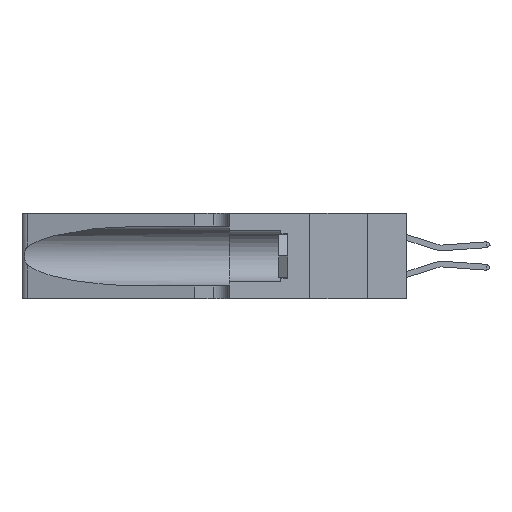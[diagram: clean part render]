
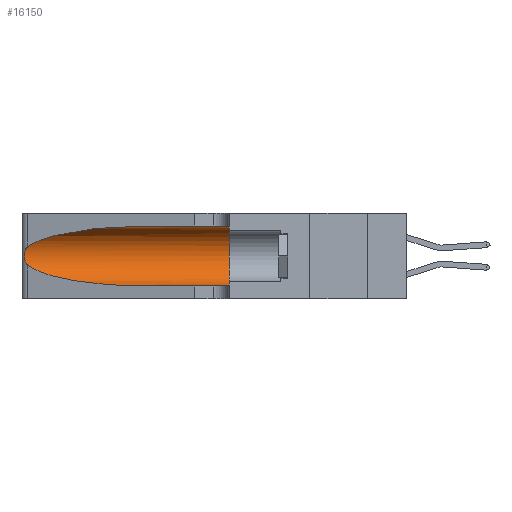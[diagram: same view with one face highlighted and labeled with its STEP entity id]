
A CAD part, left-side view. The second image highlights one B-rep face of the part: STEP entity #16150.
In plain terms, the highlighted cylindrical face has radius 3.308 mm (diameter 6.617 mm), a partial arc.
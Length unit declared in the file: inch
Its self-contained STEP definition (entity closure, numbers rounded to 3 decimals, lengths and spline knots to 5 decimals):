
#486 = ORIENTED_EDGE ( 'NONE', *, *, #4844, .T. ) ;
#889 = EDGE_CURVE ( 'NONE', #10362, #20176, #16285, .T. ) ;
#1071 = CARTESIAN_POINT ( 'NONE',  ( 0.26017, 1.23833, 0.17102 ) ) ;
#1486 = CYLINDRICAL_SURFACE ( 'NONE', #14618, 0.13025 ) ;
#2495 = CARTESIAN_POINT ( 'NONE',  ( 0.25639, 1.23184, 0.21858 ) ) ;
#2508 = CARTESIAN_POINT ( 'NONE',  ( 0.25487, 1.22718, 0.22369 ) ) ;
#2579 = VERTEX_POINT ( 'NONE', #3235 ) ;
#2772 = ORIENTED_EDGE ( 'NONE', *, *, #13080, .F. ) ;
#3235 = CARTESIAN_POINT ( 'NONE',  ( 0.25487, 1.22718, 0.14631 ) ) ;
#3304 = CARTESIAN_POINT ( 'NONE',  ( 0.1305, 0.72297, 0.31525 ) ) ;
#3445 = CARTESIAN_POINT ( 'NONE',  ( 0.1305, 1.61858, 0.31525 ) ) ;
#4004 = CARTESIAN_POINT ( 'NONE',  ( 0.25789, 1.23486, 0.15765 ) ) ;
#4145 = CARTESIAN_POINT ( 'NONE',  ( 0.25487, 1.22718, 0.22369 ) ) ;
#4205 = B_SPLINE_CURVE_WITH_KNOTS ( 'NONE', 3,
 ( #4145, #8917, #2495, #18346, #7298, #16815, #7151, #19800, #1071, #13548, #4004, #10440, #20000, #8844 ),
 .UNSPECIFIED., .F., .F.,
 ( 4, 2, 2, 2, 2, 2, 4 ),
 ( 0., 0.00027, 0.00053, 0.00107, 0.0016, 0.00187, 0.00214 ),
 .UNSPECIFIED. ) ;
#4394 = EDGE_CURVE ( 'NONE', #6285, #2579, #4205, .T. ) ;
#4625 = DIRECTION ( 'NONE',  ( 0., -1., 0. ) ) ;
#4844 = EDGE_CURVE ( 'NONE', #2579, #10362, #9988, .T. ) ;
#5320 = DIRECTION ( 'NONE',  ( 0., 1., 0. ) ) ;
#5375 = VECTOR ( 'NONE', #14432, 39.37008 ) ;
#6285 = VERTEX_POINT ( 'NONE', #2508 ) ;
#6297 =( BOUNDED_CURVE ( )  B_SPLINE_CURVE ( 3, ( #11094, #17352, #12488, #7929 ),
 .UNSPECIFIED., .F., .T. ) 
 B_SPLINE_CURVE_WITH_KNOTS ( ( 4, 4 ),
 ( 1.5708, 2.84003 ),
 .UNSPECIFIED. ) 
 CURVE ( )  GEOMETRIC_REPRESENTATION_ITEM ( )  RATIONAL_B_SPLINE_CURVE ( ( 1., 0.87, 0.87, 1. ) ) 
 REPRESENTATION_ITEM ( '' )  );
#7131 = DIRECTION ( 'NONE',  ( 0., 0., 1. ) ) ;
#7151 = CARTESIAN_POINT ( 'NONE',  ( 0.26075, 1.23896, 0.19203 ) ) ;
#7298 = CARTESIAN_POINT ( 'NONE',  ( 0.25854, 1.2359, 0.20912 ) ) ;
#7868 = CARTESIAN_POINT ( 'NONE',  ( 0.1305, 1.61858, 0.185 ) ) ;
#7929 = CARTESIAN_POINT ( 'NONE',  ( 0.25487, 1.22718, 0.22369 ) ) ;
#8217 = CARTESIAN_POINT ( 'NONE',  ( 0.1305, 0.72297, 0.05475 ) ) ;
#8728 = CARTESIAN_POINT ( 'NONE',  ( 0.25487, 1.22718, 0.14631 ) ) ;
#8844 = CARTESIAN_POINT ( 'NONE',  ( 0.25487, 1.22718, 0.14631 ) ) ;
#8917 = CARTESIAN_POINT ( 'NONE',  ( 0.25555, 1.22994, 0.2215 ) ) ;
#9678 = VERTEX_POINT ( 'NONE', #3304 ) ;
#9891 = EDGE_CURVE ( 'NONE', #9678, #10650, #12281, .T. ) ;
#9988 =( BOUNDED_CURVE ( )  B_SPLINE_CURVE ( 3, ( #8728, #14721, #14500, #8217 ),
 .UNSPECIFIED., .F., .T. ) 
 B_SPLINE_CURVE_WITH_KNOTS ( ( 4, 4 ),
 ( 3.44316, 4.71239 ),
 .UNSPECIFIED. ) 
 CURVE ( )  GEOMETRIC_REPRESENTATION_ITEM ( )  RATIONAL_B_SPLINE_CURVE ( ( 1., 0.87, 0.87, 1. ) ) 
 REPRESENTATION_ITEM ( '' )  );
#10362 = VERTEX_POINT ( 'NONE', #11983 ) ;
#10440 = CARTESIAN_POINT ( 'NONE',  ( 0.25639, 1.23186, 0.15144 ) ) ;
#10650 = VERTEX_POINT ( 'NONE', #20354 ) ;
#11094 = CARTESIAN_POINT ( 'NONE',  ( 0.1305, 0.72297, 0.31525 ) ) ;
#11978 = ORIENTED_EDGE ( 'NONE', *, *, #889, .T. ) ;
#11983 = CARTESIAN_POINT ( 'NONE',  ( 0.1305, 0.72297, 0.05475 ) ) ;
#12281 = LINE ( 'NONE', #3445, #5375 ) ;
#12450 = ORIENTED_EDGE ( 'NONE', *, *, #4394, .T. ) ;
#12488 = CARTESIAN_POINT ( 'NONE',  ( 0.2373, 1.15595, 0.28018 ) ) ;
#12538 = ORIENTED_EDGE ( 'NONE', *, *, #16108, .T. ) ;
#12758 = FACE_OUTER_BOUND ( 'NONE', #15875, .T. ) ;
#13080 = EDGE_CURVE ( 'NONE', #10650, #20176, #16396, .T. ) ;
#13085 = ORIENTED_EDGE ( 'NONE', *, *, #9891, .F. ) ;
#13168 = CARTESIAN_POINT ( 'NONE',  ( 0.1305, 0.35, 0.185 ) ) ;
#13548 = CARTESIAN_POINT ( 'NONE',  ( 0.25856, 1.23593, 0.16098 ) ) ;
#14432 = DIRECTION ( 'NONE',  ( 0., -1., 0. ) ) ;
#14500 = CARTESIAN_POINT ( 'NONE',  ( 0.18966, 0.96281, 0.05475 ) ) ;
#14618 = AXIS2_PLACEMENT_3D ( 'NONE', #7868, #4625, #15885 ) ;
#14721 = CARTESIAN_POINT ( 'NONE',  ( 0.2373, 1.15595, 0.08982 ) ) ;
#15875 = EDGE_LOOP ( 'NONE', ( #12538, #12450, #486, #11978, #2772, #13085 ) ) ;
#15885 = DIRECTION ( 'NONE',  ( 0., 0., -1. ) ) ;
#16108 = EDGE_CURVE ( 'NONE', #9678, #6285, #6297, .T. ) ;
#16150 = ADVANCED_FACE ( 'NONE', ( #12758 ), #1486, .F. ) ;
#16285 = LINE ( 'NONE', #18704, #18280 ) ;
#16323 = AXIS2_PLACEMENT_3D ( 'NONE', #13168, #5320, #7131 ) ;
#16396 = CIRCLE ( 'NONE', #16323, 0.13025 ) ;
#16428 = CARTESIAN_POINT ( 'NONE',  ( 0.1305, 0.35, 0.05475 ) ) ;
#16815 = CARTESIAN_POINT ( 'NONE',  ( 0.26018, 1.23835, 0.19895 ) ) ;
#17352 = CARTESIAN_POINT ( 'NONE',  ( 0.18966, 0.96281, 0.31525 ) ) ;
#18280 = VECTOR ( 'NONE', #20314, 39.37008 ) ;
#18346 = CARTESIAN_POINT ( 'NONE',  ( 0.25787, 1.23484, 0.2124 ) ) ;
#18704 = CARTESIAN_POINT ( 'NONE',  ( 0.1305, 1.61858, 0.05475 ) ) ;
#19800 = CARTESIAN_POINT ( 'NONE',  ( 0.26075, 1.23896, 0.178 ) ) ;
#20000 = CARTESIAN_POINT ( 'NONE',  ( 0.25555, 1.22993, 0.14849 ) ) ;
#20176 = VERTEX_POINT ( 'NONE', #16428 ) ;
#20314 = DIRECTION ( 'NONE',  ( 0., -1., 0. ) ) ;
#20354 = CARTESIAN_POINT ( 'NONE',  ( 0.1305, 0.35, 0.31525 ) ) ;
